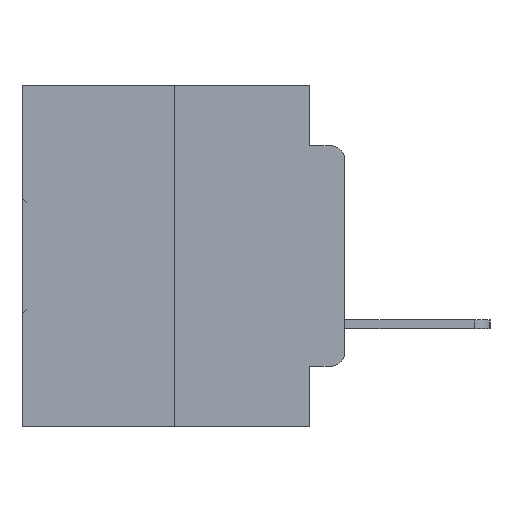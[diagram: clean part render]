
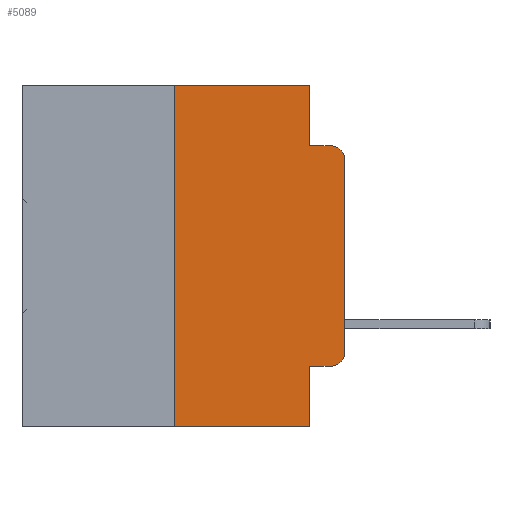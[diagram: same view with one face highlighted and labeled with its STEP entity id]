
A CAD part, left-side view. The second image highlights one B-rep face of the part: STEP entity #5089.
In plain terms, the highlighted planar face has unit normal (-1, 0, 0).
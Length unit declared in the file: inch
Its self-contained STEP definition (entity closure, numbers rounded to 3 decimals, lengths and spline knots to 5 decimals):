
#107 = LINE ( 'NONE', #13033, #6043 ) ;
#1040 = ORIENTED_EDGE ( 'NONE', *, *, #14980, .T. ) ;
#1424 = ORIENTED_EDGE ( 'NONE', *, *, #12461, .T. ) ;
#1717 = DIRECTION ( 'NONE',  ( -1., 0., 0. ) ) ;
#1839 = CIRCLE ( 'NONE', #24755, 0.02 ) ;
#3025 = ORIENTED_EDGE ( 'NONE', *, *, #4917, .F. ) ;
#3586 = CARTESIAN_POINT ( 'NONE',  ( 0., 0.25, 0. ) ) ;
#4287 = EDGE_LOOP ( 'NONE', ( #16718, #20575, #17874, #29577, #12064, #3025, #1424, #16342, #21781, #1040 ) ) ;
#4816 = CARTESIAN_POINT ( 'NONE',  ( 0., 0.051, -0.0885 ) ) ;
#4917 = EDGE_CURVE ( 'NONE', #15042, #17098, #16538, .T. ) ;
#5089 = ADVANCED_FACE ( 'NONE', ( #30888 ), #11497, .F. ) ;
#5855 = CARTESIAN_POINT ( 'NONE',  ( 0., 0.051, -0.5 ) ) ;
#6043 = VECTOR ( 'NONE', #27947, 39.37008 ) ;
#6566 = DIRECTION ( 'NONE',  ( 0., -1., 0. ) ) ;
#7085 = VECTOR ( 'NONE', #12162, 39.37008 ) ;
#7623 = VERTEX_POINT ( 'NONE', #29393 ) ;
#7876 = VECTOR ( 'NONE', #6566, 39.37008 ) ;
#8317 = EDGE_CURVE ( 'NONE', #22928, #23272, #30340, .T. ) ;
#9327 = VECTOR ( 'NONE', #14649, 39.37008 ) ;
#9457 = CARTESIAN_POINT ( 'NONE',  ( 0., 0.02, -0.4115 ) ) ;
#9950 = CARTESIAN_POINT ( 'NONE',  ( 0., 0.473, -0.5 ) ) ;
#11497 = PLANE ( 'NONE',  #21323 ) ;
#11664 = EDGE_CURVE ( 'NONE', #22928, #15086, #19662, .T. ) ;
#11943 = CARTESIAN_POINT ( 'NONE',  ( 0., 0.25, -0.5 ) ) ;
#12064 = ORIENTED_EDGE ( 'NONE', *, *, #20527, .F. ) ;
#12162 = DIRECTION ( 'NONE',  ( 0., 0., 1. ) ) ;
#12426 = DIRECTION ( 'NONE',  ( 0., -1., 0. ) ) ;
#12461 = EDGE_CURVE ( 'NONE', #15042, #23272, #21155, .T. ) ;
#12835 = VERTEX_POINT ( 'NONE', #16321 ) ;
#13013 = AXIS2_PLACEMENT_3D ( 'NONE', #16725, #1717, #19184 ) ;
#13033 = CARTESIAN_POINT ( 'NONE',  ( 0., 0.051, 0. ) ) ;
#13691 = LINE ( 'NONE', #22046, #7085 ) ;
#13933 = CARTESIAN_POINT ( 'NONE',  ( 0., 0.051, -0.4115 ) ) ;
#14081 = DIRECTION ( 'NONE',  ( -1., 0., 0. ) ) ;
#14336 = LINE ( 'NONE', #4816, #9327 ) ;
#14649 = DIRECTION ( 'NONE',  ( 0., -1., 0. ) ) ;
#14980 = EDGE_CURVE ( 'NONE', #15086, #31781, #24109, .T. ) ;
#15042 = VERTEX_POINT ( 'NONE', #11943 ) ;
#15086 = VERTEX_POINT ( 'NONE', #9457 ) ;
#15751 = VECTOR ( 'NONE', #30433, 39.37008 ) ;
#16165 = DIRECTION ( 'NONE',  ( 0., -1., 0. ) ) ;
#16321 = CARTESIAN_POINT ( 'NONE',  ( 0., 0., -0.1085 ) ) ;
#16342 = ORIENTED_EDGE ( 'NONE', *, *, #8317, .F. ) ;
#16491 = DIRECTION ( 'NONE',  ( 0., 0., -1. ) ) ;
#16538 = LINE ( 'NONE', #19239, #15751 ) ;
#16718 = ORIENTED_EDGE ( 'NONE', *, *, #20573, .T. ) ;
#16725 = CARTESIAN_POINT ( 'NONE',  ( 0., 0.02, -0.3915 ) ) ;
#17098 = VERTEX_POINT ( 'NONE', #3586 ) ;
#17874 = ORIENTED_EDGE ( 'NONE', *, *, #27304, .F. ) ;
#18969 = CARTESIAN_POINT ( 'NONE',  ( 0., 0.473, 0. ) ) ;
#19184 = DIRECTION ( 'NONE',  ( 0., 0., -1. ) ) ;
#19239 = CARTESIAN_POINT ( 'NONE',  ( 0., 0.25, 0. ) ) ;
#19662 = LINE ( 'NONE', #28672, #25510 ) ;
#20527 = EDGE_CURVE ( 'NONE', #17098, #24267, #21889, .T. ) ;
#20573 = EDGE_CURVE ( 'NONE', #31781, #12835, #13691, .T. ) ;
#20575 = ORIENTED_EDGE ( 'NONE', *, *, #22279, .T. ) ;
#21155 = LINE ( 'NONE', #9950, #26237 ) ;
#21323 = AXIS2_PLACEMENT_3D ( 'NONE', #28894, #31341, #16491 ) ;
#21781 = ORIENTED_EDGE ( 'NONE', *, *, #11664, .T. ) ;
#21889 = LINE ( 'NONE', #18969, #7876 ) ;
#22046 = CARTESIAN_POINT ( 'NONE',  ( 0., 0., 0. ) ) ;
#22212 = CARTESIAN_POINT ( 'NONE',  ( 0., 0.051, 0. ) ) ;
#22279 = EDGE_CURVE ( 'NONE', #12835, #29543, #1839, .T. ) ;
#22928 = VERTEX_POINT ( 'NONE', #13933 ) ;
#23272 = VERTEX_POINT ( 'NONE', #5855 ) ;
#23739 = VECTOR ( 'NONE', #24708, 39.37008 ) ;
#24109 = CIRCLE ( 'NONE', #13013, 0.02 ) ;
#24267 = VERTEX_POINT ( 'NONE', #24978 ) ;
#24708 = DIRECTION ( 'NONE',  ( 0., 0., -1. ) ) ;
#24755 = AXIS2_PLACEMENT_3D ( 'NONE', #29020, #14081, #31448 ) ;
#24978 = CARTESIAN_POINT ( 'NONE',  ( 0., 0.051, 0. ) ) ;
#25510 = VECTOR ( 'NONE', #16165, 39.37008 ) ;
#26237 = VECTOR ( 'NONE', #12426, 39.37008 ) ;
#26462 = CARTESIAN_POINT ( 'NONE',  ( 0., 0.02, -0.0885 ) ) ;
#27304 = EDGE_CURVE ( 'NONE', #7623, #29543, #14336, .T. ) ;
#27338 = CARTESIAN_POINT ( 'NONE',  ( 0., 0., -0.3915 ) ) ;
#27947 = DIRECTION ( 'NONE',  ( 0., 0., -1. ) ) ;
#28672 = CARTESIAN_POINT ( 'NONE',  ( 0., 0.051, -0.4115 ) ) ;
#28894 = CARTESIAN_POINT ( 'NONE',  ( 0., 0.473, 0. ) ) ;
#29020 = CARTESIAN_POINT ( 'NONE',  ( 0., 0.02, -0.1085 ) ) ;
#29393 = CARTESIAN_POINT ( 'NONE',  ( 0., 0.051, -0.0885 ) ) ;
#29543 = VERTEX_POINT ( 'NONE', #26462 ) ;
#29577 = ORIENTED_EDGE ( 'NONE', *, *, #30588, .F. ) ;
#30340 = LINE ( 'NONE', #22212, #23739 ) ;
#30433 = DIRECTION ( 'NONE',  ( 0., 0., 1. ) ) ;
#30588 = EDGE_CURVE ( 'NONE', #24267, #7623, #107, .T. ) ;
#30888 = FACE_OUTER_BOUND ( 'NONE', #4287, .T. ) ;
#31341 = DIRECTION ( 'NONE',  ( 1., 0., 0. ) ) ;
#31448 = DIRECTION ( 'NONE',  ( 0., 0., -1. ) ) ;
#31781 = VERTEX_POINT ( 'NONE', #27338 ) ;
